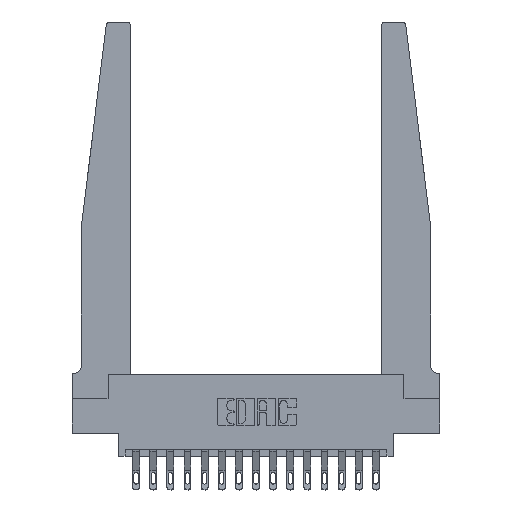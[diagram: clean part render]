
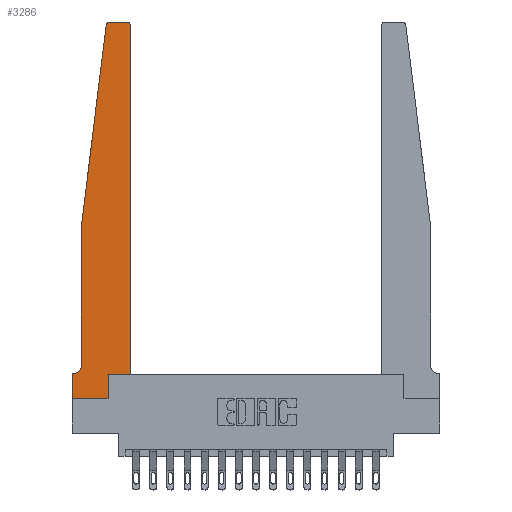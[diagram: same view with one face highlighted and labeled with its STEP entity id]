
A CAD part, top view. The second image highlights one B-rep face of the part: STEP entity #3286.
In plain terms, the highlighted planar face has unit normal (0, 0, 1).
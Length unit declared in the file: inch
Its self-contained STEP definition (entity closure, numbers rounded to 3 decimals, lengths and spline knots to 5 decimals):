
#65 = LINE ( 'NONE', #4511, #14865 ) ;
#259 = LINE ( 'NONE', #16297, #13021 ) ;
#267 = LINE ( 'NONE', #17951, #16192 ) ;
#432 = ORIENTED_EDGE ( 'NONE', *, *, #13786, .T. ) ;
#448 = VERTEX_POINT ( 'NONE', #17446 ) ;
#667 = VECTOR ( 'NONE', #1696, 39.37008 ) ;
#799 = EDGE_CURVE ( 'NONE', #7277, #448, #3697, .T. ) ;
#802 = VERTEX_POINT ( 'NONE', #14042 ) ;
#960 = CIRCLE ( 'NONE', #11760, 0.05 ) ;
#982 = DIRECTION ( 'NONE',  ( 0., 0., -1. ) ) ;
#994 = CARTESIAN_POINT ( 'NONE',  ( 0., 0.1875, 0.37 ) ) ;
#1178 = LINE ( 'NONE', #10320, #5763 ) ;
#1696 = DIRECTION ( 'NONE',  ( 0., -1., 0. ) ) ;
#1949 = EDGE_CURVE ( 'NONE', #13414, #5443, #14824, .T. ) ;
#2304 = CARTESIAN_POINT ( 'NONE',  ( 0., 0., 0.37 ) ) ;
#2536 = EDGE_CURVE ( 'NONE', #448, #8266, #3387, .T. ) ;
#2575 = EDGE_CURVE ( 'NONE', #5005, #7373, #960, .T. ) ;
#2917 = AXIS2_PLACEMENT_3D ( 'NONE', #16654, #17812, #15205 ) ;
#3024 = EDGE_CURVE ( 'NONE', #7373, #4557, #65, .T. ) ;
#3214 = CARTESIAN_POINT ( 'NONE',  ( 0.2605, 0.18, 0.37 ) ) ;
#3286 = ADVANCED_FACE ( 'NONE', ( #14221 ), #15678, .T. ) ;
#3387 = LINE ( 'NONE', #12488, #5268 ) ;
#3449 = DIRECTION ( 'NONE',  ( -1., 0., 0. ) ) ;
#3626 = VERTEX_POINT ( 'NONE', #2304 ) ;
#3697 = LINE ( 'NONE', #9616, #13877 ) ;
#3796 = CARTESIAN_POINT ( 'NONE',  ( 0.015, 0.1875, 0.37 ) ) ;
#4008 = CARTESIAN_POINT ( 'NONE',  ( 0.2605, 0., 0.37 ) ) ;
#4205 = VERTEX_POINT ( 'NONE', #4008 ) ;
#4293 = EDGE_CURVE ( 'NONE', #4557, #3626, #11851, .T. ) ;
#4397 = ORIENTED_EDGE ( 'NONE', *, *, #7606, .T. ) ;
#4511 = CARTESIAN_POINT ( 'NONE',  ( 0.065, 0.1875, 0.37 ) ) ;
#4557 = VERTEX_POINT ( 'NONE', #17157 ) ;
#5005 = VERTEX_POINT ( 'NONE', #16158 ) ;
#5114 = EDGE_CURVE ( 'NONE', #7177, #13414, #12454, .T. ) ;
#5268 = VECTOR ( 'NONE', #10941, 39.37008 ) ;
#5443 = VERTEX_POINT ( 'NONE', #7516 ) ;
#5763 = VECTOR ( 'NONE', #7730, 39.37008 ) ;
#6898 = ORIENTED_EDGE ( 'NONE', *, *, #16864, .T. ) ;
#7177 = VERTEX_POINT ( 'NONE', #17831 ) ;
#7277 = VERTEX_POINT ( 'NONE', #3214 ) ;
#7373 = VERTEX_POINT ( 'NONE', #3796 ) ;
#7516 = CARTESIAN_POINT ( 'NONE',  ( 0.24675, 2.72367, 0.37 ) ) ;
#7525 = DIRECTION ( 'NONE',  ( 0., 0., 1. ) ) ;
#7606 = EDGE_CURVE ( 'NONE', #8266, #7177, #16836, .T. ) ;
#7611 = CARTESIAN_POINT ( 'NONE',  ( 0., 0., 0.37 ) ) ;
#7730 = DIRECTION ( 'NONE',  ( 0., 1., 0. ) ) ;
#7750 = AXIS2_PLACEMENT_3D ( 'NONE', #10134, #7525, #13402 ) ;
#7822 = VECTOR ( 'NONE', #3449, 39.37008 ) ;
#8266 = VERTEX_POINT ( 'NONE', #17290 ) ;
#8671 = VECTOR ( 'NONE', #8977, 39.37008 ) ;
#8924 = ORIENTED_EDGE ( 'NONE', *, *, #12654, .T. ) ;
#8977 = DIRECTION ( 'NONE',  ( -0.122, -0.992, 0. ) ) ;
#9108 = ORIENTED_EDGE ( 'NONE', *, *, #2575, .T. ) ;
#9616 = CARTESIAN_POINT ( 'NONE',  ( 0.425, 0.18, 0.37 ) ) ;
#10134 = CARTESIAN_POINT ( 'NONE',  ( 0.27653, 2.72, 0.37 ) ) ;
#10304 = EDGE_CURVE ( 'NONE', #802, #5005, #259, .T. ) ;
#10320 = CARTESIAN_POINT ( 'NONE',  ( 0.2605, 0.18, 0.37 ) ) ;
#10411 = LINE ( 'NONE', #16304, #8671 ) ;
#10539 = ORIENTED_EDGE ( 'NONE', *, *, #3024, .T. ) ;
#10662 = ORIENTED_EDGE ( 'NONE', *, *, #10304, .T. ) ;
#10710 = ORIENTED_EDGE ( 'NONE', *, *, #5114, .T. ) ;
#10788 = ORIENTED_EDGE ( 'NONE', *, *, #799, .T. ) ;
#10941 = DIRECTION ( 'NONE',  ( 0., 1., 0. ) ) ;
#11413 = CARTESIAN_POINT ( 'NONE',  ( 0.015, 0.2375, 0.37 ) ) ;
#11473 = ORIENTED_EDGE ( 'NONE', *, *, #1949, .T. ) ;
#11760 = AXIS2_PLACEMENT_3D ( 'NONE', #11413, #982, #13047 ) ;
#11851 = LINE ( 'NONE', #7611, #667 ) ;
#12454 = LINE ( 'NONE', #15536, #7822 ) ;
#12488 = CARTESIAN_POINT ( 'NONE',  ( 0.425, 0.18, 0.37 ) ) ;
#12654 = EDGE_CURVE ( 'NONE', #3626, #4205, #267, .T. ) ;
#13021 = VECTOR ( 'NONE', #14849, 39.37008 ) ;
#13047 = DIRECTION ( 'NONE',  ( -1., 0., 0. ) ) ;
#13402 = DIRECTION ( 'NONE',  ( 1., 0., 0. ) ) ;
#13414 = VERTEX_POINT ( 'NONE', #15264 ) ;
#13502 = DIRECTION ( 'NONE',  ( -1., 0., 0. ) ) ;
#13767 = DIRECTION ( 'NONE',  ( 1., 0., 0. ) ) ;
#13786 = EDGE_CURVE ( 'NONE', #5443, #802, #10411, .T. ) ;
#13877 = VECTOR ( 'NONE', #13767, 39.37008 ) ;
#14042 = CARTESIAN_POINT ( 'NONE',  ( 0.065, 1.25, 0.37 ) ) ;
#14221 = FACE_OUTER_BOUND ( 'NONE', #16972, .T. ) ;
#14250 = AXIS2_PLACEMENT_3D ( 'NONE', #994, #18769, #17227 ) ;
#14824 = CIRCLE ( 'NONE', #7750, 0.03 ) ;
#14849 = DIRECTION ( 'NONE',  ( 0., -1., 0. ) ) ;
#14865 = VECTOR ( 'NONE', #13502, 39.37008 ) ;
#15205 = DIRECTION ( 'NONE',  ( 1., 0., 0. ) ) ;
#15218 = ORIENTED_EDGE ( 'NONE', *, *, #4293, .T. ) ;
#15264 = CARTESIAN_POINT ( 'NONE',  ( 0.27653, 2.75, 0.37 ) ) ;
#15536 = CARTESIAN_POINT ( 'NONE',  ( 0.25, 2.75, 0.37 ) ) ;
#15678 = PLANE ( 'NONE',  #14250 ) ;
#16158 = CARTESIAN_POINT ( 'NONE',  ( 0.065, 0.2375, 0.37 ) ) ;
#16192 = VECTOR ( 'NONE', #17846, 39.37008 ) ;
#16297 = CARTESIAN_POINT ( 'NONE',  ( 0.065, 1.25, 0.37 ) ) ;
#16304 = CARTESIAN_POINT ( 'NONE',  ( 0.065, 1.25, 0.37 ) ) ;
#16654 = CARTESIAN_POINT ( 'NONE',  ( 0.395, 2.72, 0.37 ) ) ;
#16836 = CIRCLE ( 'NONE', #2917, 0.03 ) ;
#16864 = EDGE_CURVE ( 'NONE', #4205, #7277, #1178, .T. ) ;
#16972 = EDGE_LOOP ( 'NONE', ( #10710, #11473, #432, #10662, #9108, #10539, #15218, #8924, #6898, #10788, #18801, #4397 ) ) ;
#17157 = CARTESIAN_POINT ( 'NONE',  ( 0., 0.1875, 0.37 ) ) ;
#17227 = DIRECTION ( 'NONE',  ( 1., 0., 0. ) ) ;
#17290 = CARTESIAN_POINT ( 'NONE',  ( 0.425, 2.72, 0.37 ) ) ;
#17446 = CARTESIAN_POINT ( 'NONE',  ( 0.425, 0.18, 0.37 ) ) ;
#17812 = DIRECTION ( 'NONE',  ( 0., 0., 1. ) ) ;
#17831 = CARTESIAN_POINT ( 'NONE',  ( 0.395, 2.75, 0.37 ) ) ;
#17846 = DIRECTION ( 'NONE',  ( 1., 0., 0. ) ) ;
#17951 = CARTESIAN_POINT ( 'NONE',  ( 0., 0., 0.37 ) ) ;
#18769 = DIRECTION ( 'NONE',  ( 0., 0., 1. ) ) ;
#18801 = ORIENTED_EDGE ( 'NONE', *, *, #2536, .T. ) ;
